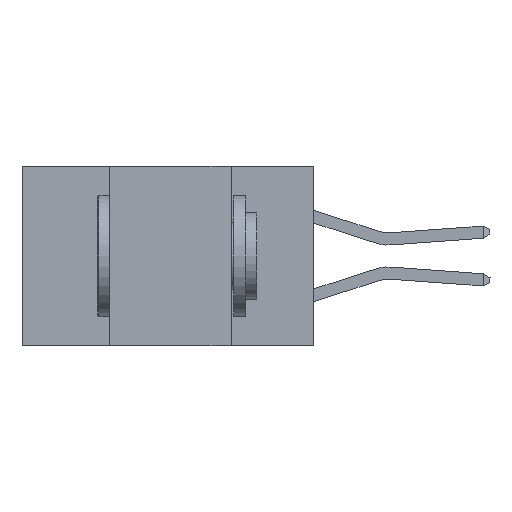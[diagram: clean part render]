
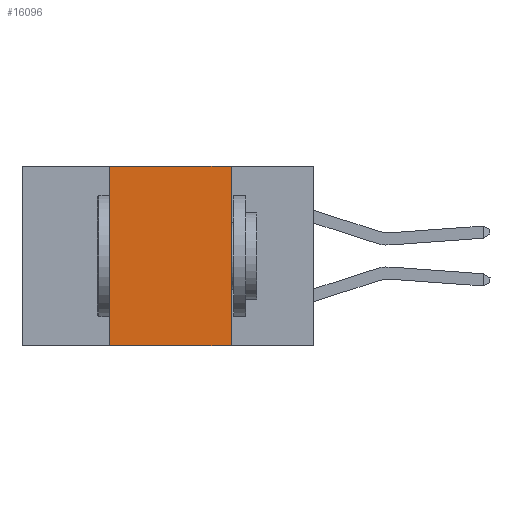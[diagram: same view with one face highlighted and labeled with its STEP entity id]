
A CAD part, left-side view. The second image highlights one B-rep face of the part: STEP entity #16096.
In plain terms, the highlighted planar face has unit normal (-1, 0, 0).
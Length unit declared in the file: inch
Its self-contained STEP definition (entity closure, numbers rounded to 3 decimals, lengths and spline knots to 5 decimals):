
#133 = VECTOR ( 'NONE', #1476, 39.37008 ) ;
#265 = CARTESIAN_POINT ( 'NONE',  ( 0., 0.17, 0. ) ) ;
#465 = LINE ( 'NONE', #9694, #8940 ) ;
#1257 = VERTEX_POINT ( 'NONE', #16012 ) ;
#1476 = DIRECTION ( 'NONE',  ( 0., 0., -1. ) ) ;
#1622 = ORIENTED_EDGE ( 'NONE', *, *, #18057, .T. ) ;
#2597 = CARTESIAN_POINT ( 'NONE',  ( 0., 0.6, 0. ) ) ;
#2881 = CARTESIAN_POINT ( 'NONE',  ( 0., 0.6, -0.37 ) ) ;
#2966 = LINE ( 'NONE', #16439, #18437 ) ;
#3651 = EDGE_LOOP ( 'NONE', ( #16804, #5451, #9581, #1622 ) ) ;
#4262 = DIRECTION ( 'NONE',  ( 0., 0., -1. ) ) ;
#4992 = VECTOR ( 'NONE', #17904, 39.37008 ) ;
#5148 = CARTESIAN_POINT ( 'NONE',  ( 0., 0.42, -0.37 ) ) ;
#5451 = ORIENTED_EDGE ( 'NONE', *, *, #5973, .F. ) ;
#5973 = EDGE_CURVE ( 'NONE', #1257, #7683, #465, .T. ) ;
#7497 = EDGE_CURVE ( 'NONE', #7683, #19233, #9129, .T. ) ;
#7683 = VERTEX_POINT ( 'NONE', #265 ) ;
#8940 = VECTOR ( 'NONE', #9579, 39.37008 ) ;
#9129 = LINE ( 'NONE', #9401, #133 ) ;
#9151 = LINE ( 'NONE', #2881, #4992 ) ;
#9401 = CARTESIAN_POINT ( 'NONE',  ( 0., 0.17, 0. ) ) ;
#9579 = DIRECTION ( 'NONE',  ( 0., -1., 0. ) ) ;
#9581 = ORIENTED_EDGE ( 'NONE', *, *, #14441, .F. ) ;
#9694 = CARTESIAN_POINT ( 'NONE',  ( 0., 0.6, 0. ) ) ;
#10777 = DIRECTION ( 'NONE',  ( 0., 0., 1. ) ) ;
#12016 = PLANE ( 'NONE',  #18843 ) ;
#13456 = DIRECTION ( 'NONE',  ( 1., 0., 0. ) ) ;
#14441 = EDGE_CURVE ( 'NONE', #17054, #1257, #2966, .T. ) ;
#16012 = CARTESIAN_POINT ( 'NONE',  ( 0., 0.42, 0. ) ) ;
#16096 = ADVANCED_FACE ( 'NONE', ( #19247 ), #12016, .F. ) ;
#16439 = CARTESIAN_POINT ( 'NONE',  ( 0., 0.42, 0. ) ) ;
#16804 = ORIENTED_EDGE ( 'NONE', *, *, #7497, .F. ) ;
#16974 = CARTESIAN_POINT ( 'NONE',  ( 0., 0.17, -0.37 ) ) ;
#17054 = VERTEX_POINT ( 'NONE', #5148 ) ;
#17904 = DIRECTION ( 'NONE',  ( 0., -1., 0. ) ) ;
#18057 = EDGE_CURVE ( 'NONE', #17054, #19233, #9151, .T. ) ;
#18437 = VECTOR ( 'NONE', #10777, 39.37008 ) ;
#18843 = AXIS2_PLACEMENT_3D ( 'NONE', #2597, #13456, #4262 ) ;
#19233 = VERTEX_POINT ( 'NONE', #16974 ) ;
#19247 = FACE_OUTER_BOUND ( 'NONE', #3651, .T. ) ;
